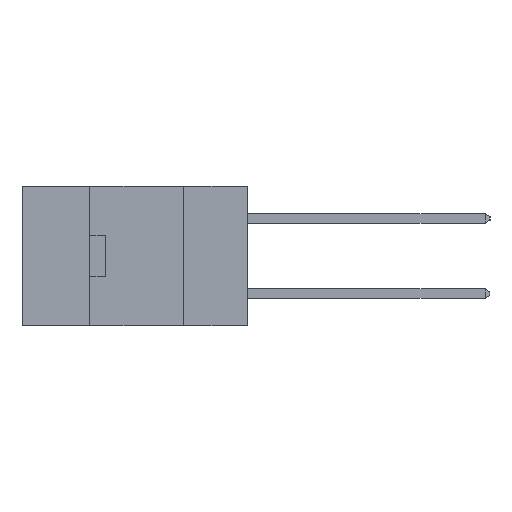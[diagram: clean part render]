
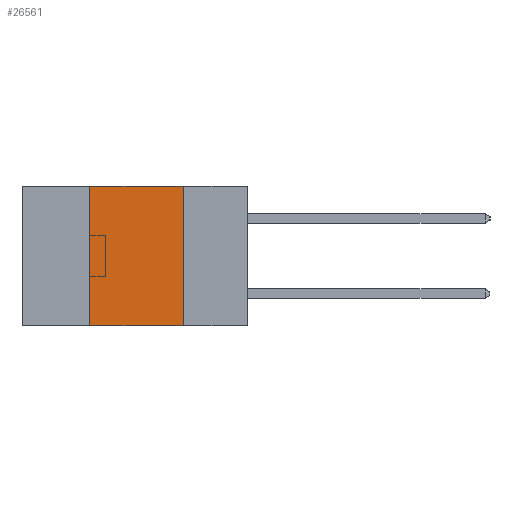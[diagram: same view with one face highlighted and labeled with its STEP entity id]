
A CAD part, left-side view. The second image highlights one B-rep face of the part: STEP entity #26561.
In plain terms, the highlighted planar face has unit normal (-1, 0, 0).
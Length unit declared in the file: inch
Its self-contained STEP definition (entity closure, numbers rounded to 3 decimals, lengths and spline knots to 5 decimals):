
#1329 = VECTOR ( 'NONE', #5126, 39.37008 ) ;
#1620 = CARTESIAN_POINT ( 'NONE',  ( 0., 0.42, -0.37 ) ) ;
#1802 = CARTESIAN_POINT ( 'NONE',  ( 0., 0.17, -0.37 ) ) ;
#2507 = CARTESIAN_POINT ( 'NONE',  ( 0., 0.17, -0.37 ) ) ;
#2951 = CARTESIAN_POINT ( 'NONE',  ( 0., 0.6, -0.37 ) ) ;
#3734 = DIRECTION ( 'NONE',  ( 0., 0., 1. ) ) ;
#3922 = DIRECTION ( 'NONE',  ( 0., 0., -1. ) ) ;
#5126 = DIRECTION ( 'NONE',  ( 0., -1., 0. ) ) ;
#5142 = CARTESIAN_POINT ( 'NONE',  ( 0., 0.6, 0. ) ) ;
#5616 = ORIENTED_EDGE ( 'NONE', *, *, #23979, .F. ) ;
#6302 = ORIENTED_EDGE ( 'NONE', *, *, #22542, .F. ) ;
#6472 = VERTEX_POINT ( 'NONE', #10928 ) ;
#7203 = CARTESIAN_POINT ( 'NONE',  ( 0., 0.42, 0. ) ) ;
#7324 = EDGE_LOOP ( 'NONE', ( #5616, #6302, #18523, #7684 ) ) ;
#7326 = DIRECTION ( 'NONE',  ( 0., 0., -1. ) ) ;
#7684 = ORIENTED_EDGE ( 'NONE', *, *, #16781, .T. ) ;
#10648 = AXIS2_PLACEMENT_3D ( 'NONE', #5142, #20283, #7326 ) ;
#10928 = CARTESIAN_POINT ( 'NONE',  ( 0., 0.17, 0. ) ) ;
#11585 = LINE ( 'NONE', #1620, #23070 ) ;
#12826 = LINE ( 'NONE', #2951, #1329 ) ;
#14241 = VECTOR ( 'NONE', #3922, 39.37008 ) ;
#16366 = VECTOR ( 'NONE', #23395, 39.37008 ) ;
#16781 = EDGE_CURVE ( 'NONE', #18088, #26417, #12826, .T. ) ;
#18088 = VERTEX_POINT ( 'NONE', #20122 ) ;
#18428 = FACE_OUTER_BOUND ( 'NONE', #7324, .T. ) ;
#18523 = ORIENTED_EDGE ( 'NONE', *, *, #21085, .F. ) ;
#18988 = CARTESIAN_POINT ( 'NONE',  ( 0., 0.6, 0. ) ) ;
#20122 = CARTESIAN_POINT ( 'NONE',  ( 0., 0.42, -0.37 ) ) ;
#20283 = DIRECTION ( 'NONE',  ( 1., 0., 0. ) ) ;
#21085 = EDGE_CURVE ( 'NONE', #18088, #27573, #11585, .T. ) ;
#22103 = LINE ( 'NONE', #18988, #16366 ) ;
#22356 = PLANE ( 'NONE',  #10648 ) ;
#22542 = EDGE_CURVE ( 'NONE', #27573, #6472, #22103, .T. ) ;
#23070 = VECTOR ( 'NONE', #3734, 39.37008 ) ;
#23395 = DIRECTION ( 'NONE',  ( 0., -1., 0. ) ) ;
#23979 = EDGE_CURVE ( 'NONE', #6472, #26417, #25672, .T. ) ;
#25672 = LINE ( 'NONE', #1802, #14241 ) ;
#26417 = VERTEX_POINT ( 'NONE', #2507 ) ;
#26561 = ADVANCED_FACE ( 'NONE', ( #18428 ), #22356, .F. ) ;
#27573 = VERTEX_POINT ( 'NONE', #7203 ) ;
